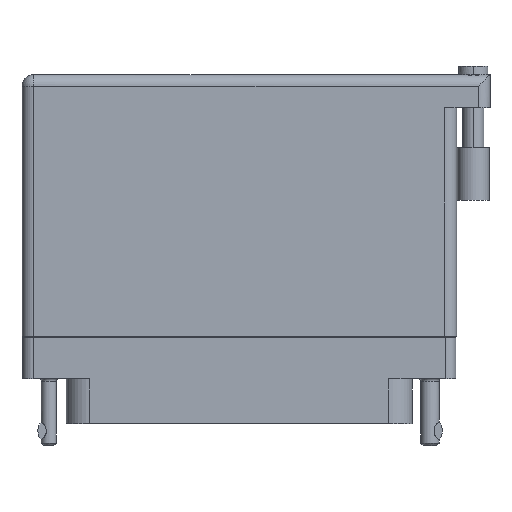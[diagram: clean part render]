
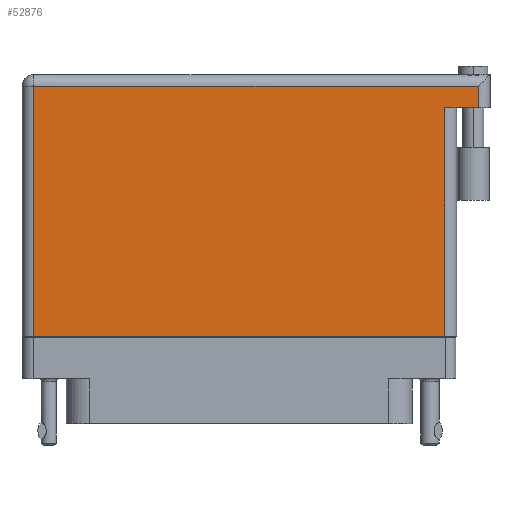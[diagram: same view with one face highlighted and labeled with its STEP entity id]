
A CAD part, front view. The second image highlights one B-rep face of the part: STEP entity #52876.
In plain terms, the highlighted face is planar.
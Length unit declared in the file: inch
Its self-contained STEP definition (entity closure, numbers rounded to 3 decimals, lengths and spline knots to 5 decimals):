
#949 = AXIS2_PLACEMENT_3D ( 'NONE', #22973, #4869, #27880 ) ;
#2319 = LINE ( 'NONE', #57777, #38316 ) ;
#3140 = VERTEX_POINT ( 'NONE', #32742 ) ;
#4469 = EDGE_CURVE ( 'NONE', #10916, #25058, #53055, .T. ) ;
#4869 = DIRECTION ( 'NONE',  ( 0., 0., -1. ) ) ;
#10916 = VERTEX_POINT ( 'NONE', #51206 ) ;
#11947 = CARTESIAN_POINT ( 'NONE',  ( 1.43, 1.466, 0.4495 ) ) ;
#12511 = ORIENTED_EDGE ( 'NONE', *, *, #57569, .T. ) ;
#12779 = VERTEX_POINT ( 'NONE', #12863 ) ;
#12863 = CARTESIAN_POINT ( 'NONE',  ( 1.43, 1.269, 0.4495 ) ) ;
#15873 = VECTOR ( 'NONE', #21367, 39.37008 ) ;
#17307 = LINE ( 'NONE', #11947, #15873 ) ;
#17856 = VECTOR ( 'NONE', #52273, 39.37008 ) ;
#17907 = ORIENTED_EDGE ( 'NONE', *, *, #24258, .F. ) ;
#19131 = ORIENTED_EDGE ( 'NONE', *, *, #22800, .T. ) ;
#21367 = DIRECTION ( 'NONE',  ( 0., 1., 0. ) ) ;
#21879 = LINE ( 'NONE', #56638, #57899 ) ;
#22800 = EDGE_CURVE ( 'NONE', #3140, #25409, #33995, .T. ) ;
#22973 = CARTESIAN_POINT ( 'NONE',  ( -1.3, 1.466, 0.4495 ) ) ;
#23182 = PLANE ( 'NONE',  #949 ) ;
#24258 = EDGE_CURVE ( 'NONE', #12779, #25409, #2319, .T. ) ;
#25058 = VERTEX_POINT ( 'NONE', #49839 ) ;
#25409 = VERTEX_POINT ( 'NONE', #39130 ) ;
#27880 = DIRECTION ( 'NONE',  ( -1., 0., 0. ) ) ;
#28087 = LINE ( 'NONE', #49889, #32463 ) ;
#32463 = VECTOR ( 'NONE', #54172, 39.37008 ) ;
#32742 = CARTESIAN_POINT ( 'NONE',  ( 1.23, -0.1, 0.4495 ) ) ;
#33995 = LINE ( 'NONE', #47192, #17856 ) ;
#34376 = DIRECTION ( 'NONE',  ( -1., 0., 0. ) ) ;
#38312 = CARTESIAN_POINT ( 'NONE',  ( -1.3, 1.396, 0.4495 ) ) ;
#38316 = VECTOR ( 'NONE', #34376, 39.37008 ) ;
#39130 = CARTESIAN_POINT ( 'NONE',  ( 1.23, 1.269, 0.4495 ) ) ;
#41791 = ORIENTED_EDGE ( 'NONE', *, *, #52216, .T. ) ;
#47192 = CARTESIAN_POINT ( 'NONE',  ( 1.23, 1.269, 0.4495 ) ) ;
#49839 = CARTESIAN_POINT ( 'NONE',  ( -1.23, 1.396, 0.4495 ) ) ;
#49889 = CARTESIAN_POINT ( 'NONE',  ( -1.3, -0.1, 0.4495 ) ) ;
#51206 = CARTESIAN_POINT ( 'NONE',  ( 1.43, 1.396, 0.4495 ) ) ;
#51546 = VECTOR ( 'NONE', #52030, 39.37008 ) ;
#51893 = DIRECTION ( 'NONE',  ( 0., -1., 0. ) ) ;
#51902 = EDGE_LOOP ( 'NONE', ( #41791, #19131, #17907, #12511, #60657, #57614 ) ) ;
#52030 = DIRECTION ( 'NONE',  ( -1., 0., 0. ) ) ;
#52216 = EDGE_CURVE ( 'NONE', #55529, #3140, #28087, .T. ) ;
#52273 = DIRECTION ( 'NONE',  ( 0., 1., 0. ) ) ;
#52876 = ADVANCED_FACE ( 'NONE', ( #58869 ), #23182, .F. ) ;
#53055 = LINE ( 'NONE', #38312, #51546 ) ;
#54172 = DIRECTION ( 'NONE',  ( 1., 0., 0. ) ) ;
#55529 = VERTEX_POINT ( 'NONE', #58619 ) ;
#56638 = CARTESIAN_POINT ( 'NONE',  ( -1.23, -0.1, 0.4495 ) ) ;
#57569 = EDGE_CURVE ( 'NONE', #12779, #10916, #17307, .T. ) ;
#57614 = ORIENTED_EDGE ( 'NONE', *, *, #58817, .T. ) ;
#57777 = CARTESIAN_POINT ( 'NONE',  ( 1.5, 1.269, 0.4495 ) ) ;
#57899 = VECTOR ( 'NONE', #51893, 39.37008 ) ;
#58619 = CARTESIAN_POINT ( 'NONE',  ( -1.23, -0.1, 0.4495 ) ) ;
#58817 = EDGE_CURVE ( 'NONE', #25058, #55529, #21879, .T. ) ;
#58869 = FACE_OUTER_BOUND ( 'NONE', #51902, .T. ) ;
#60657 = ORIENTED_EDGE ( 'NONE', *, *, #4469, .T. ) ;
